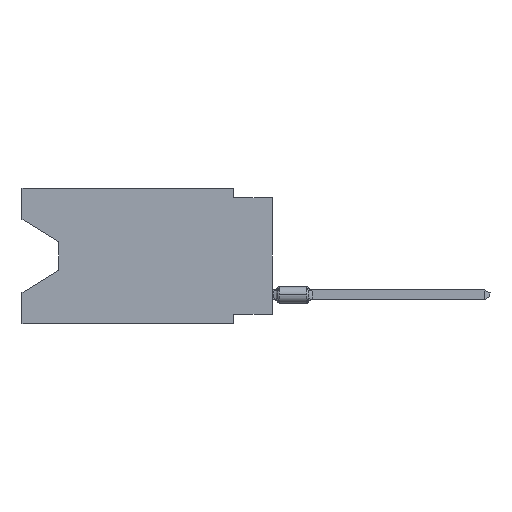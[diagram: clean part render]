
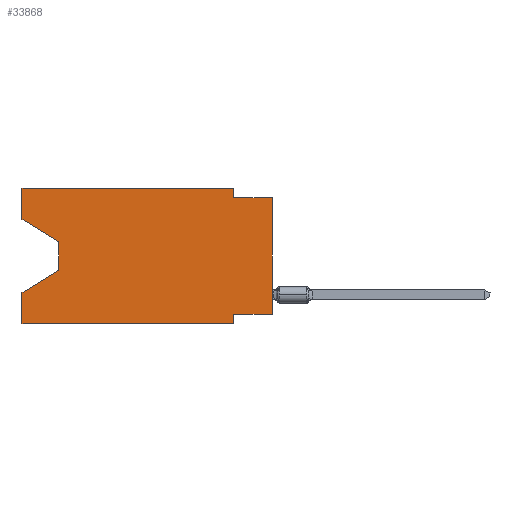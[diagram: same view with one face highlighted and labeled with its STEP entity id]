
A CAD part, left-side view. The second image highlights one B-rep face of the part: STEP entity #33868.
In plain terms, the highlighted planar face has unit normal (-1, 0, 0).
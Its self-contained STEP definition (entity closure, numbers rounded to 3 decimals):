
#245 = DIRECTION ( 'NONE',  ( 0., 1., 0. ) ) ;
#315 = CARTESIAN_POINT ( 'NONE',  ( 0., 16.383, 0. ) ) ;
#509 = DIRECTION ( 'NONE',  ( 0., -1., 0. ) ) ;
#618 = CARTESIAN_POINT ( 'NONE',  ( 0., 16.383, -8.89 ) ) ;
#689 = CARTESIAN_POINT ( 'NONE',  ( 0., 0., -8.255 ) ) ;
#859 = CARTESIAN_POINT ( 'NONE',  ( 0., 16.383, -2.038 ) ) ;
#1696 = ORIENTED_EDGE ( 'NONE', *, *, #18963, .F. ) ;
#1900 = CARTESIAN_POINT ( 'NONE',  ( 0., 16.383, -6.852 ) ) ;
#2106 = DIRECTION ( 'NONE',  ( 0., -0.855, -0.519 ) ) ;
#2385 = VERTEX_POINT ( 'NONE', #27856 ) ;
#3808 = LINE ( 'NONE', #26573, #23909 ) ;
#3952 = CARTESIAN_POINT ( 'NONE',  ( 0., 2.54, 0. ) ) ;
#4388 = EDGE_CURVE ( 'NONE', #24715, #31358, #33975, .T. ) ;
#4581 = VECTOR ( 'NONE', #2106, 1000. ) ;
#4848 = CARTESIAN_POINT ( 'NONE',  ( 0., 13.97, -5.385 ) ) ;
#6465 = VERTEX_POINT ( 'NONE', #859 ) ;
#6925 = VERTEX_POINT ( 'NONE', #33709 ) ;
#7659 = CARTESIAN_POINT ( 'NONE',  ( 0., 16.383, 0. ) ) ;
#7834 = DIRECTION ( 'NONE',  ( 0., 0., -1. ) ) ;
#8922 = CARTESIAN_POINT ( 'NONE',  ( 0., 16.383, 0. ) ) ;
#9371 = VECTOR ( 'NONE', #245, 1000. ) ;
#10389 = VECTOR ( 'NONE', #41450, 1000. ) ;
#10526 = ORIENTED_EDGE ( 'NONE', *, *, #22805, .F. ) ;
#10778 = VERTEX_POINT ( 'NONE', #14842 ) ;
#11373 = DIRECTION ( 'NONE',  ( 0., 0., 1. ) ) ;
#11494 = CARTESIAN_POINT ( 'NONE',  ( 0., 16.383, 0. ) ) ;
#11739 = VECTOR ( 'NONE', #24158, 1000. ) ;
#12439 = ORIENTED_EDGE ( 'NONE', *, *, #19668, .F. ) ;
#12494 = LINE ( 'NONE', #29045, #4581 ) ;
#13318 = VECTOR ( 'NONE', #38426, 1000. ) ;
#14003 = EDGE_LOOP ( 'NONE', ( #28438, #32760, #24012, #1696, #14380, #22729, #12439, #15340, #10526, #28615, #26398, #35952 ) ) ;
#14324 = VECTOR ( 'NONE', #7834, 1000. ) ;
#14325 = LINE ( 'NONE', #618, #10389 ) ;
#14380 = ORIENTED_EDGE ( 'NONE', *, *, #42727, .T. ) ;
#14397 = EDGE_CURVE ( 'NONE', #6465, #28459, #21861, .T. ) ;
#14654 = CARTESIAN_POINT ( 'NONE',  ( 0., 13.97, -3.505 ) ) ;
#14842 = CARTESIAN_POINT ( 'NONE',  ( 0., 2.54, -8.89 ) ) ;
#15340 = ORIENTED_EDGE ( 'NONE', *, *, #22738, .T. ) ;
#15461 = VECTOR ( 'NONE', #509, 1000. ) ;
#15634 = EDGE_CURVE ( 'NONE', #19241, #42856, #35098, .T. ) ;
#16393 = FACE_OUTER_BOUND ( 'NONE', #14003, .T. ) ;
#17763 = LINE ( 'NONE', #315, #11739 ) ;
#18870 = EDGE_CURVE ( 'NONE', #2385, #10778, #34123, .T. ) ;
#18963 = EDGE_CURVE ( 'NONE', #22775, #42856, #39176, .T. ) ;
#19241 = VERTEX_POINT ( 'NONE', #30326 ) ;
#19668 = EDGE_CURVE ( 'NONE', #36940, #2385, #23866, .T. ) ;
#20167 = LINE ( 'NONE', #33620, #15461 ) ;
#21861 = LINE ( 'NONE', #11494, #13318 ) ;
#22729 = ORIENTED_EDGE ( 'NONE', *, *, #18870, .F. ) ;
#22738 = EDGE_CURVE ( 'NONE', #36940, #38644, #3808, .T. ) ;
#22775 = VERTEX_POINT ( 'NONE', #27002 ) ;
#22805 = EDGE_CURVE ( 'NONE', #31358, #38644, #20167, .T. ) ;
#23866 = LINE ( 'NONE', #689, #9371 ) ;
#23909 = VECTOR ( 'NONE', #23910, 1000. ) ;
#23910 = DIRECTION ( 'NONE',  ( 0., 0., 1. ) ) ;
#24012 = ORIENTED_EDGE ( 'NONE', *, *, #15634, .T. ) ;
#24158 = DIRECTION ( 'NONE',  ( 0., -1., 0. ) ) ;
#24165 = EDGE_CURVE ( 'NONE', #6925, #19241, #27882, .T. ) ;
#24715 = VERTEX_POINT ( 'NONE', #33500 ) ;
#24851 = VECTOR ( 'NONE', #11373, 1000. ) ;
#26148 = VECTOR ( 'NONE', #28105, 1000. ) ;
#26398 = ORIENTED_EDGE ( 'NONE', *, *, #30015, .F. ) ;
#26573 = CARTESIAN_POINT ( 'NONE',  ( 0., 0., 0. ) ) ;
#26761 = DIRECTION ( 'NONE',  ( 1., 0., 0. ) ) ;
#27002 = CARTESIAN_POINT ( 'NONE',  ( 0., 16.383, -8.89 ) ) ;
#27071 = CARTESIAN_POINT ( 'NONE',  ( 0., 2.54, -8.89 ) ) ;
#27330 = VECTOR ( 'NONE', #28025, 1000. ) ;
#27522 = VECTOR ( 'NONE', #42365, 1000. ) ;
#27856 = CARTESIAN_POINT ( 'NONE',  ( 0., 2.54, -8.255 ) ) ;
#27882 = LINE ( 'NONE', #14654, #26148 ) ;
#28025 = DIRECTION ( 'NONE',  ( 0., 0., -1. ) ) ;
#28105 = DIRECTION ( 'NONE',  ( 0., 0., -1. ) ) ;
#28438 = ORIENTED_EDGE ( 'NONE', *, *, #40039, .T. ) ;
#28459 = VERTEX_POINT ( 'NONE', #7659 ) ;
#28615 = ORIENTED_EDGE ( 'NONE', *, *, #4388, .F. ) ;
#29045 = CARTESIAN_POINT ( 'NONE',  ( 0., 16.383, -2.038 ) ) ;
#30015 = EDGE_CURVE ( 'NONE', #28459, #24715, #17763, .T. ) ;
#30065 = PLANE ( 'NONE',  #34115 ) ;
#30072 = CARTESIAN_POINT ( 'NONE',  ( 0., 0., -0.635 ) ) ;
#30326 = CARTESIAN_POINT ( 'NONE',  ( 0., 13.97, -5.385 ) ) ;
#31358 = VERTEX_POINT ( 'NONE', #40192 ) ;
#32760 = ORIENTED_EDGE ( 'NONE', *, *, #24165, .T. ) ;
#33500 = CARTESIAN_POINT ( 'NONE',  ( 0., 2.54, 0. ) ) ;
#33620 = CARTESIAN_POINT ( 'NONE',  ( 0., 0., -0.635 ) ) ;
#33709 = CARTESIAN_POINT ( 'NONE',  ( 0., 13.97, -3.505 ) ) ;
#33868 = ADVANCED_FACE ( 'NONE', ( #16393 ), #30065, .F. ) ;
#33975 = LINE ( 'NONE', #3952, #27330 ) ;
#34115 = AXIS2_PLACEMENT_3D ( 'NONE', #36918, #26761, #36245 ) ;
#34123 = LINE ( 'NONE', #27071, #14324 ) ;
#35098 = LINE ( 'NONE', #4848, #27522 ) ;
#35952 = ORIENTED_EDGE ( 'NONE', *, *, #14397, .F. ) ;
#36245 = DIRECTION ( 'NONE',  ( 0., 0., -1. ) ) ;
#36918 = CARTESIAN_POINT ( 'NONE',  ( 0., 16.383, 0. ) ) ;
#36940 = VERTEX_POINT ( 'NONE', #40648 ) ;
#38426 = DIRECTION ( 'NONE',  ( 0., 0., 1. ) ) ;
#38644 = VERTEX_POINT ( 'NONE', #30072 ) ;
#39176 = LINE ( 'NONE', #8922, #24851 ) ;
#40039 = EDGE_CURVE ( 'NONE', #6465, #6925, #12494, .T. ) ;
#40192 = CARTESIAN_POINT ( 'NONE',  ( 0., 2.54, -0.635 ) ) ;
#40648 = CARTESIAN_POINT ( 'NONE',  ( 0., 0., -8.255 ) ) ;
#41450 = DIRECTION ( 'NONE',  ( 0., -1., 0. ) ) ;
#42365 = DIRECTION ( 'NONE',  ( 0., 0.855, -0.519 ) ) ;
#42727 = EDGE_CURVE ( 'NONE', #22775, #10778, #14325, .T. ) ;
#42856 = VERTEX_POINT ( 'NONE', #1900 ) ;
